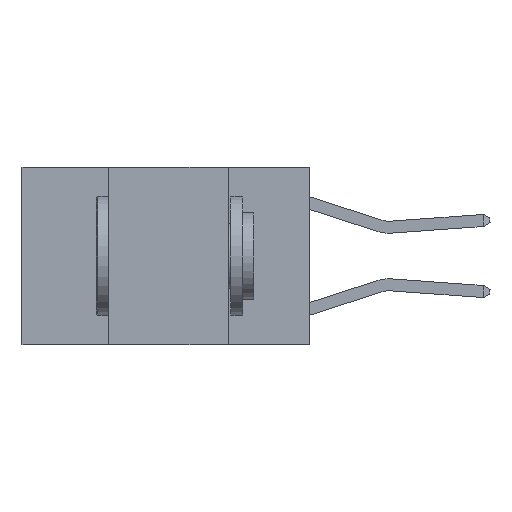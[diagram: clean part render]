
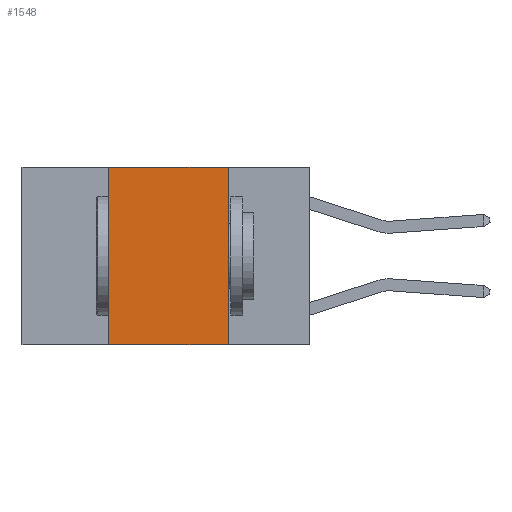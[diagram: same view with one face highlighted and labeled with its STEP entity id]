
A CAD part, left-side view. The second image highlights one B-rep face of the part: STEP entity #1548.
In plain terms, the highlighted planar face has unit normal (-1, 0, 0).
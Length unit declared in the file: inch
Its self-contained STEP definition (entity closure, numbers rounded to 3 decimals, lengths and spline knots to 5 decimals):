
#412 = CARTESIAN_POINT ( 'NONE',  ( 0., 0.42, 0. ) ) ;
#479 = DIRECTION ( 'NONE',  ( 0., 0., -1. ) ) ;
#1053 = DIRECTION ( 'NONE',  ( 0., 0., 1. ) ) ;
#1548 = ADVANCED_FACE ( 'NONE', ( #12497 ), #17522, .F. ) ;
#1895 = VERTEX_POINT ( 'NONE', #6671 ) ;
#3355 = ORIENTED_EDGE ( 'NONE', *, *, #6110, .T. ) ;
#4152 = ORIENTED_EDGE ( 'NONE', *, *, #13798, .F. ) ;
#4201 = ORIENTED_EDGE ( 'NONE', *, *, #20780, .F. ) ;
#5007 = LINE ( 'NONE', #19967, #7887 ) ;
#5999 = DIRECTION ( 'NONE',  ( 0., 0., -1. ) ) ;
#6110 = EDGE_CURVE ( 'NONE', #15942, #9232, #5007, .T. ) ;
#6671 = CARTESIAN_POINT ( 'NONE',  ( 0., 0.17, 0. ) ) ;
#7330 = LINE ( 'NONE', #15935, #13529 ) ;
#7407 = CARTESIAN_POINT ( 'NONE',  ( 0., 0.17, -0.37 ) ) ;
#7887 = VECTOR ( 'NONE', #11680, 39.37008 ) ;
#9232 = VERTEX_POINT ( 'NONE', #7407 ) ;
#10893 = LINE ( 'NONE', #12372, #13048 ) ;
#11166 = CARTESIAN_POINT ( 'NONE',  ( 0., 0.42, 0. ) ) ;
#11680 = DIRECTION ( 'NONE',  ( 0., -1., 0. ) ) ;
#12372 = CARTESIAN_POINT ( 'NONE',  ( 0., 0.6, 0. ) ) ;
#12497 = FACE_OUTER_BOUND ( 'NONE', #21251, .T. ) ;
#12872 = LINE ( 'NONE', #11166, #13857 ) ;
#13048 = VECTOR ( 'NONE', #19193, 39.37008 ) ;
#13529 = VECTOR ( 'NONE', #5999, 39.37008 ) ;
#13798 = EDGE_CURVE ( 'NONE', #15942, #15721, #12872, .T. ) ;
#13857 = VECTOR ( 'NONE', #1053, 39.37008 ) ;
#15083 = CARTESIAN_POINT ( 'NONE',  ( 0., 0.42, -0.37 ) ) ;
#15721 = VERTEX_POINT ( 'NONE', #412 ) ;
#15935 = CARTESIAN_POINT ( 'NONE',  ( 0., 0.17, 0. ) ) ;
#15942 = VERTEX_POINT ( 'NONE', #15083 ) ;
#17522 = PLANE ( 'NONE',  #19794 ) ;
#18065 = EDGE_CURVE ( 'NONE', #15721, #1895, #10893, .T. ) ;
#19193 = DIRECTION ( 'NONE',  ( 0., -1., 0. ) ) ;
#19794 = AXIS2_PLACEMENT_3D ( 'NONE', #20476, #20877, #479 ) ;
#19967 = CARTESIAN_POINT ( 'NONE',  ( 0., 0.6, -0.37 ) ) ;
#20476 = CARTESIAN_POINT ( 'NONE',  ( 0., 0.6, 0. ) ) ;
#20780 = EDGE_CURVE ( 'NONE', #1895, #9232, #7330, .T. ) ;
#20824 = ORIENTED_EDGE ( 'NONE', *, *, #18065, .F. ) ;
#20877 = DIRECTION ( 'NONE',  ( 1., 0., 0. ) ) ;
#21251 = EDGE_LOOP ( 'NONE', ( #4201, #20824, #4152, #3355 ) ) ;
